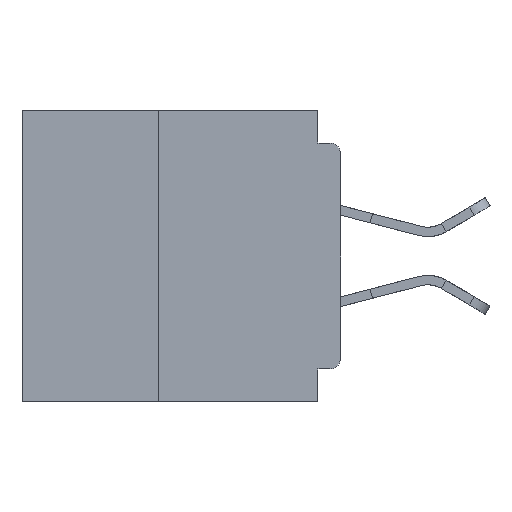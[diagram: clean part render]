
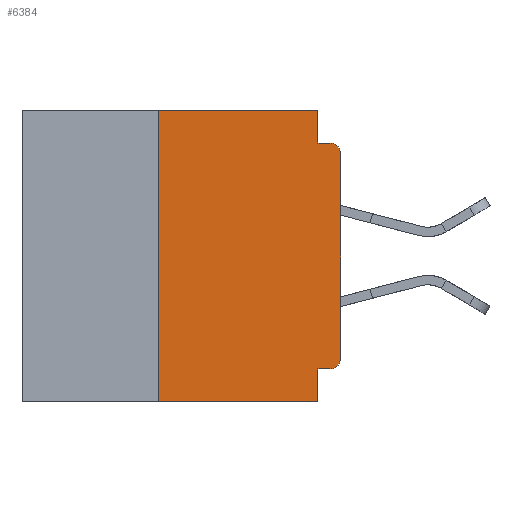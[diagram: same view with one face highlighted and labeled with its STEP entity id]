
A CAD part, left-side view. The second image highlights one B-rep face of the part: STEP entity #6384.
In plain terms, the highlighted planar face has unit normal (-1, 0, 0).
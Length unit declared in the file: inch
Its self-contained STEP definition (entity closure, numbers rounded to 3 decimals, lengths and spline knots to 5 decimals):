
#40 = DIRECTION ( 'NONE',  ( 1., 0., 0. ) ) ;
#261 = AXIS2_PLACEMENT_3D ( 'NONE', #21875, #40, #22020 ) ;
#632 = AXIS2_PLACEMENT_3D ( 'NONE', #39179, #20443, #1621 ) ;
#745 = LINE ( 'NONE', #9511, #9052 ) ;
#1179 = CARTESIAN_POINT ( 'NONE',  ( 0., 0.015, -0.34 ) ) ;
#1621 = DIRECTION ( 'NONE',  ( 0., 0., -1. ) ) ;
#1804 = VERTEX_POINT ( 'NONE', #6936 ) ;
#1917 = EDGE_CURVE ( 'NONE', #20201, #25301, #3998, .T. ) ;
#1921 = VERTEX_POINT ( 'NONE', #25803 ) ;
#2023 = ORIENTED_EDGE ( 'NONE', *, *, #7703, .T. ) ;
#2157 = EDGE_CURVE ( 'NONE', #25301, #33681, #17286, .T. ) ;
#3392 = EDGE_LOOP ( 'NONE', ( #2023, #22780, #38412, #21531, #6420, #13178, #34637, #12632, #11774, #31125 ) ) ;
#3998 = LINE ( 'NONE', #32323, #12383 ) ;
#4289 = DIRECTION ( 'NONE',  ( 0., 0., -1. ) ) ;
#4932 = LINE ( 'NONE', #22477, #36368 ) ;
#5438 = CARTESIAN_POINT ( 'NONE',  ( 0., 0.25, 0. ) ) ;
#6373 = CARTESIAN_POINT ( 'NONE',  ( 0., 0., 0. ) ) ;
#6384 = ADVANCED_FACE ( 'NONE', ( #19845 ), #18882, .F. ) ;
#6420 = ORIENTED_EDGE ( 'NONE', *, *, #33920, .F. ) ;
#6780 = DIRECTION ( 'NONE',  ( 0., -1., 0. ) ) ;
#6936 = CARTESIAN_POINT ( 'NONE',  ( 0., 0.015, -0.045 ) ) ;
#7195 = LINE ( 'NONE', #34187, #22938 ) ;
#7703 = EDGE_CURVE ( 'NONE', #35174, #22383, #15309, .T. ) ;
#7751 = EDGE_CURVE ( 'NONE', #17859, #1804, #4932, .T. ) ;
#8226 = DIRECTION ( 'NONE',  ( 0., -1., 0. ) ) ;
#9052 = VECTOR ( 'NONE', #31476, 39.37008 ) ;
#9511 = CARTESIAN_POINT ( 'NONE',  ( 0., 0.25, -0.4 ) ) ;
#9891 = VECTOR ( 'NONE', #28599, 39.37008 ) ;
#10199 = CARTESIAN_POINT ( 'NONE',  ( 0., 0., -0.34 ) ) ;
#10292 = EDGE_CURVE ( 'NONE', #22383, #1804, #18300, .T. ) ;
#11774 = ORIENTED_EDGE ( 'NONE', *, *, #1917, .F. ) ;
#12383 = VECTOR ( 'NONE', #33299, 39.37008 ) ;
#12632 = ORIENTED_EDGE ( 'NONE', *, *, #2157, .F. ) ;
#13178 = ORIENTED_EDGE ( 'NONE', *, *, #23350, .F. ) ;
#13194 = DIRECTION ( 'NONE',  ( 0., 0., -1. ) ) ;
#13586 = CIRCLE ( 'NONE', #14946, 0.015 ) ;
#13671 = LINE ( 'NONE', #23905, #21039 ) ;
#14412 = EDGE_CURVE ( 'NONE', #20201, #35174, #13586, .T. ) ;
#14946 = AXIS2_PLACEMENT_3D ( 'NONE', #1179, #23149, #4289 ) ;
#15309 = LINE ( 'NONE', #6373, #22688 ) ;
#15890 = DIRECTION ( 'NONE',  ( 0., 0., 1. ) ) ;
#16621 = CARTESIAN_POINT ( 'NONE',  ( 0., 0., -0.06 ) ) ;
#17286 = LINE ( 'NONE', #27064, #9891 ) ;
#17433 = CARTESIAN_POINT ( 'NONE',  ( 0., 0.25, -0.4 ) ) ;
#17859 = VERTEX_POINT ( 'NONE', #18936 ) ;
#18300 = CIRCLE ( 'NONE', #632, 0.015 ) ;
#18609 = VECTOR ( 'NONE', #13194, 39.37008 ) ;
#18882 = PLANE ( 'NONE',  #261 ) ;
#18936 = CARTESIAN_POINT ( 'NONE',  ( 0., 0.031, -0.045 ) ) ;
#19845 = FACE_OUTER_BOUND ( 'NONE', #3392, .T. ) ;
#20201 = VERTEX_POINT ( 'NONE', #30078 ) ;
#20443 = DIRECTION ( 'NONE',  ( -1., 0., 0. ) ) ;
#21039 = VECTOR ( 'NONE', #8226, 39.37008 ) ;
#21531 = ORIENTED_EDGE ( 'NONE', *, *, #40289, .F. ) ;
#21875 = CARTESIAN_POINT ( 'NONE',  ( 0., 0.437, 0. ) ) ;
#22020 = DIRECTION ( 'NONE',  ( 0., 0., -1. ) ) ;
#22383 = VERTEX_POINT ( 'NONE', #16621 ) ;
#22477 = CARTESIAN_POINT ( 'NONE',  ( 0., 0., -0.045 ) ) ;
#22688 = VECTOR ( 'NONE', #15890, 39.37008 ) ;
#22780 = ORIENTED_EDGE ( 'NONE', *, *, #10292, .T. ) ;
#22938 = VECTOR ( 'NONE', #28084, 39.37008 ) ;
#23002 = CARTESIAN_POINT ( 'NONE',  ( 0., 0.031, -0.355 ) ) ;
#23149 = DIRECTION ( 'NONE',  ( -1., 0., 0. ) ) ;
#23350 = EDGE_CURVE ( 'NONE', #37845, #35004, #745, .T. ) ;
#23905 = CARTESIAN_POINT ( 'NONE',  ( 0., 0.437, -0.4 ) ) ;
#25301 = VERTEX_POINT ( 'NONE', #23002 ) ;
#25803 = CARTESIAN_POINT ( 'NONE',  ( 0., 0.031, 0. ) ) ;
#26892 = CARTESIAN_POINT ( 'NONE',  ( 0., 0.031, -0.4 ) ) ;
#27064 = CARTESIAN_POINT ( 'NONE',  ( 0., 0.031, -0.4 ) ) ;
#28084 = DIRECTION ( 'NONE',  ( 0., -1., 0. ) ) ;
#28599 = DIRECTION ( 'NONE',  ( 0., 0., -1. ) ) ;
#30078 = CARTESIAN_POINT ( 'NONE',  ( 0., 0.015, -0.355 ) ) ;
#31125 = ORIENTED_EDGE ( 'NONE', *, *, #14412, .T. ) ;
#31476 = DIRECTION ( 'NONE',  ( 0., 0., 1. ) ) ;
#31965 = CARTESIAN_POINT ( 'NONE',  ( 0., 0.031, 0. ) ) ;
#32323 = CARTESIAN_POINT ( 'NONE',  ( 0., 0., -0.355 ) ) ;
#33097 = EDGE_CURVE ( 'NONE', #37845, #33681, #13671, .T. ) ;
#33299 = DIRECTION ( 'NONE',  ( 0., 1., 0. ) ) ;
#33681 = VERTEX_POINT ( 'NONE', #26892 ) ;
#33920 = EDGE_CURVE ( 'NONE', #35004, #1921, #7195, .T. ) ;
#34187 = CARTESIAN_POINT ( 'NONE',  ( 0., 0.437, 0. ) ) ;
#34637 = ORIENTED_EDGE ( 'NONE', *, *, #33097, .T. ) ;
#35004 = VERTEX_POINT ( 'NONE', #5438 ) ;
#35174 = VERTEX_POINT ( 'NONE', #10199 ) ;
#35230 = LINE ( 'NONE', #31965, #18609 ) ;
#36368 = VECTOR ( 'NONE', #6780, 39.37008 ) ;
#37845 = VERTEX_POINT ( 'NONE', #17433 ) ;
#38412 = ORIENTED_EDGE ( 'NONE', *, *, #7751, .F. ) ;
#39179 = CARTESIAN_POINT ( 'NONE',  ( 0., 0.015, -0.06 ) ) ;
#40289 = EDGE_CURVE ( 'NONE', #1921, #17859, #35230, .T. ) ;
